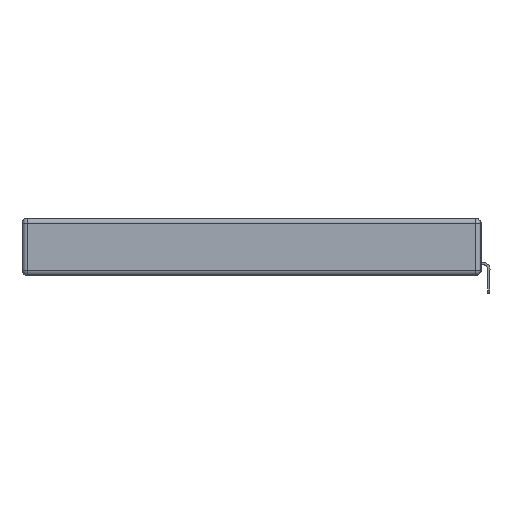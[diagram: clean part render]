
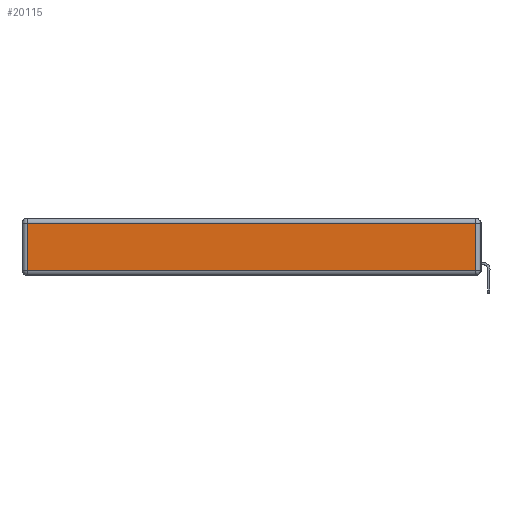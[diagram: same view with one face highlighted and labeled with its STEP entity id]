
A CAD part, left-side view. The second image highlights one B-rep face of the part: STEP entity #20115.
In plain terms, the highlighted planar face has unit normal (-1, 0, 0).
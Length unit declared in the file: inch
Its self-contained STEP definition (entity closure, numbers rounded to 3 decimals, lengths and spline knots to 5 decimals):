
#194 = EDGE_CURVE ( 'NONE', #23058, #13703, #14612, .T. ) ;
#1072 = CARTESIAN_POINT ( 'NONE',  ( 0., 0.03, -0.343 ) ) ;
#1775 = CARTESIAN_POINT ( 'NONE',  ( 0., 2.72, -0.343 ) ) ;
#1989 = CARTESIAN_POINT ( 'NONE',  ( 0., 0., -0.313 ) ) ;
#2079 = EDGE_CURVE ( 'NONE', #13831, #22451, #12392, .T. ) ;
#3264 = ORIENTED_EDGE ( 'NONE', *, *, #3688, .T. ) ;
#3688 = EDGE_CURVE ( 'NONE', #22451, #23058, #7203, .T. ) ;
#4185 = CARTESIAN_POINT ( 'NONE',  ( 0., 2.72, -0.313 ) ) ;
#4656 = DIRECTION ( 'NONE',  ( -1., 0., 0. ) ) ;
#4944 = VECTOR ( 'NONE', #6626, 39.37008 ) ;
#5715 = AXIS2_PLACEMENT_3D ( 'NONE', #17915, #4656, #19838 ) ;
#6626 = DIRECTION ( 'NONE',  ( 0., 1., 0. ) ) ;
#7203 = LINE ( 'NONE', #1072, #7802 ) ;
#7802 = VECTOR ( 'NONE', #24224, 39.37008 ) ;
#9704 = VECTOR ( 'NONE', #13164, 39.37008 ) ;
#10864 = CARTESIAN_POINT ( 'NONE',  ( 0., 0.03, -0.03 ) ) ;
#11503 = DIRECTION ( 'NONE',  ( 0., -1., 0. ) ) ;
#12392 = LINE ( 'NONE', #1989, #17519 ) ;
#13164 = DIRECTION ( 'NONE',  ( 0., 0., -1. ) ) ;
#13703 = VERTEX_POINT ( 'NONE', #17358 ) ;
#13831 = VERTEX_POINT ( 'NONE', #4185 ) ;
#14201 = PLANE ( 'NONE',  #5715 ) ;
#14326 = CARTESIAN_POINT ( 'NONE',  ( 0., 2.75, -0.03 ) ) ;
#14612 = LINE ( 'NONE', #14326, #4944 ) ;
#16661 = LINE ( 'NONE', #1775, #9704 ) ;
#17358 = CARTESIAN_POINT ( 'NONE',  ( 0., 2.72, -0.03 ) ) ;
#17519 = VECTOR ( 'NONE', #11503, 39.37008 ) ;
#17915 = CARTESIAN_POINT ( 'NONE',  ( 0., 0., -0.343 ) ) ;
#18819 = EDGE_CURVE ( 'NONE', #13703, #13831, #16661, .T. ) ;
#19838 = DIRECTION ( 'NONE',  ( 0., 0., 1. ) ) ;
#19877 = FACE_OUTER_BOUND ( 'NONE', #23088, .T. ) ;
#20115 = ADVANCED_FACE ( 'NONE', ( #19877 ), #14201, .T. ) ;
#21469 = ORIENTED_EDGE ( 'NONE', *, *, #194, .T. ) ;
#21657 = ORIENTED_EDGE ( 'NONE', *, *, #18819, .T. ) ;
#22182 = CARTESIAN_POINT ( 'NONE',  ( 0., 0.03, -0.313 ) ) ;
#22451 = VERTEX_POINT ( 'NONE', #22182 ) ;
#23058 = VERTEX_POINT ( 'NONE', #10864 ) ;
#23088 = EDGE_LOOP ( 'NONE', ( #23991, #3264, #21469, #21657 ) ) ;
#23991 = ORIENTED_EDGE ( 'NONE', *, *, #2079, .T. ) ;
#24224 = DIRECTION ( 'NONE',  ( 0., 0., 1. ) ) ;
